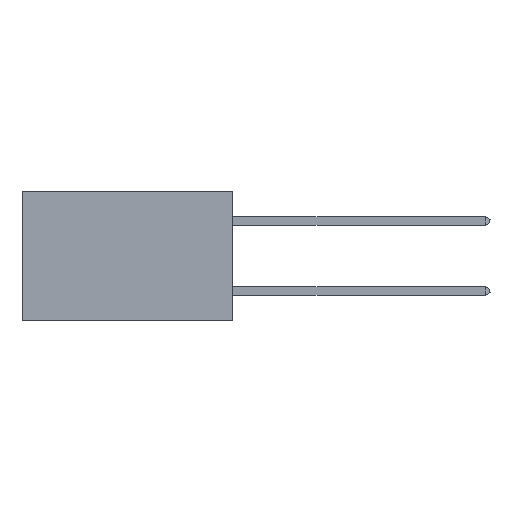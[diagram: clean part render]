
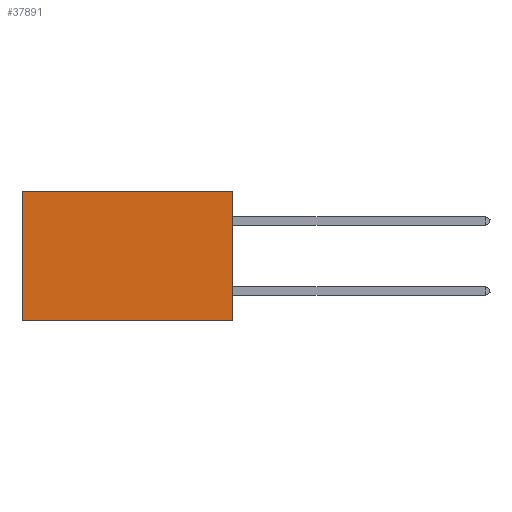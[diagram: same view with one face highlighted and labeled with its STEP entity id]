
A CAD part, left-side view. The second image highlights one B-rep face of the part: STEP entity #37891.
In plain terms, the highlighted planar face has unit normal (-1, 0, 0).
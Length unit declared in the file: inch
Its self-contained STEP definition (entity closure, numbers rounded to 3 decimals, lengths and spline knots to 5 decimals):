
#608 = LINE ( 'NONE', #30163, #37176 ) ;
#751 = EDGE_CURVE ( 'NONE', #18254, #17414, #7274, .T. ) ;
#4599 = CARTESIAN_POINT ( 'NONE',  ( 0.2875, 0.6, 0. ) ) ;
#5853 = DIRECTION ( 'NONE',  ( 0., 0., -1. ) ) ;
#7274 = LINE ( 'NONE', #4599, #35420 ) ;
#8632 = LINE ( 'NONE', #8978, #26352 ) ;
#8978 = CARTESIAN_POINT ( 'NONE',  ( 0.2875, 0., 0. ) ) ;
#9217 = FACE_OUTER_BOUND ( 'NONE', #27938, .T. ) ;
#10338 = EDGE_CURVE ( 'NONE', #30031, #18254, #608, .T. ) ;
#10840 = CARTESIAN_POINT ( 'NONE',  ( 0.2875, 0., 0. ) ) ;
#11043 = DIRECTION ( 'NONE',  ( 0., 1., 0. ) ) ;
#12284 = DIRECTION ( 'NONE',  ( 0., 0., -1. ) ) ;
#13038 = ORIENTED_EDGE ( 'NONE', *, *, #25468, .F. ) ;
#17414 = VERTEX_POINT ( 'NONE', #33761 ) ;
#18043 = CARTESIAN_POINT ( 'NONE',  ( 0.2875, 0., -0.37 ) ) ;
#18254 = VERTEX_POINT ( 'NONE', #41801 ) ;
#18590 = AXIS2_PLACEMENT_3D ( 'NONE', #36692, #33302, #12284 ) ;
#19693 = DIRECTION ( 'NONE',  ( 0., 0., -1. ) ) ;
#20136 = ORIENTED_EDGE ( 'NONE', *, *, #10338, .T. ) ;
#25468 = EDGE_CURVE ( 'NONE', #42197, #17414, #26618, .T. ) ;
#26352 = VECTOR ( 'NONE', #19693, 39.37008 ) ;
#26618 = LINE ( 'NONE', #18043, #43012 ) ;
#26660 = DIRECTION ( 'NONE',  ( 0., 1., 0. ) ) ;
#27938 = EDGE_LOOP ( 'NONE', ( #39342, #13038, #37717, #20136 ) ) ;
#29625 = CARTESIAN_POINT ( 'NONE',  ( 0.2875, 0., -0.37 ) ) ;
#29783 = PLANE ( 'NONE',  #18590 ) ;
#30031 = VERTEX_POINT ( 'NONE', #10840 ) ;
#30163 = CARTESIAN_POINT ( 'NONE',  ( 0.2875, 0., 0. ) ) ;
#32327 = EDGE_CURVE ( 'NONE', #30031, #42197, #8632, .T. ) ;
#33302 = DIRECTION ( 'NONE',  ( 1., 0., 0. ) ) ;
#33761 = CARTESIAN_POINT ( 'NONE',  ( 0.2875, 0.6, -0.37 ) ) ;
#35420 = VECTOR ( 'NONE', #5853, 39.37008 ) ;
#36692 = CARTESIAN_POINT ( 'NONE',  ( 0.2875, 0., 0. ) ) ;
#37176 = VECTOR ( 'NONE', #26660, 39.37008 ) ;
#37717 = ORIENTED_EDGE ( 'NONE', *, *, #32327, .F. ) ;
#37891 = ADVANCED_FACE ( 'NONE', ( #9217 ), #29783, .F. ) ;
#39342 = ORIENTED_EDGE ( 'NONE', *, *, #751, .T. ) ;
#41801 = CARTESIAN_POINT ( 'NONE',  ( 0.2875, 0.6, 0. ) ) ;
#42197 = VERTEX_POINT ( 'NONE', #29625 ) ;
#43012 = VECTOR ( 'NONE', #11043, 39.37008 ) ;
